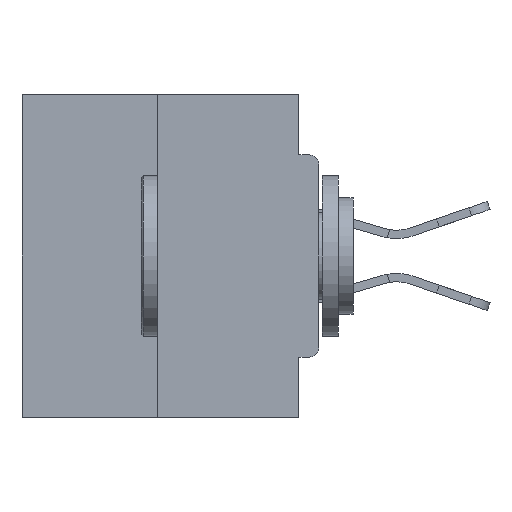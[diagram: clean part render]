
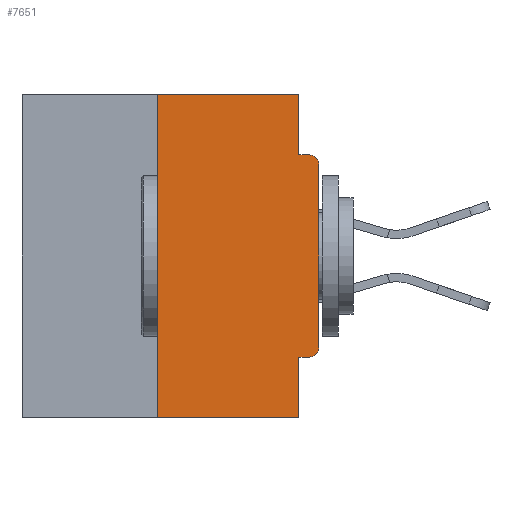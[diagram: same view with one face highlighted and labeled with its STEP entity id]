
A CAD part, left-side view. The second image highlights one B-rep face of the part: STEP entity #7651.
In plain terms, the highlighted planar face has unit normal (-1, 0, 0).
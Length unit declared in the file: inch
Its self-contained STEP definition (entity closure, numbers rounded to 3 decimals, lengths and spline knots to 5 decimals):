
#301 = FACE_OUTER_BOUND ( 'NONE', #33683, .T. ) ;
#410 = ORIENTED_EDGE ( 'NONE', *, *, #1086, .T. ) ;
#1086 = EDGE_CURVE ( 'NONE', #6244, #31713, #26061, .T. ) ;
#1896 = CARTESIAN_POINT ( 'NONE',  ( 0., 0., -0.0935 ) ) ;
#2441 = VERTEX_POINT ( 'NONE', #15004 ) ;
#2601 = CARTESIAN_POINT ( 'NONE',  ( 0., 0.015, -0.3915 ) ) ;
#3044 = DIRECTION ( 'NONE',  ( 0., 0., -1. ) ) ;
#3548 = CARTESIAN_POINT ( 'NONE',  ( 0., 0.46, -0.5 ) ) ;
#3959 = VECTOR ( 'NONE', #20573, 39.37008 ) ;
#4343 = VERTEX_POINT ( 'NONE', #19120 ) ;
#4525 = EDGE_CURVE ( 'NONE', #5938, #28625, #33759, .T. ) ;
#4541 = ORIENTED_EDGE ( 'NONE', *, *, #6182, .F. ) ;
#4792 = ORIENTED_EDGE ( 'NONE', *, *, #29375, .T. ) ;
#4930 = DIRECTION ( 'NONE',  ( 0., -1., 0. ) ) ;
#5081 = CARTESIAN_POINT ( 'NONE',  ( 0., 0., -0.4065 ) ) ;
#5479 = DIRECTION ( 'NONE',  ( 0., 0., 1. ) ) ;
#5938 = VERTEX_POINT ( 'NONE', #21699 ) ;
#6148 = ORIENTED_EDGE ( 'NONE', *, *, #4525, .F. ) ;
#6182 = EDGE_CURVE ( 'NONE', #21148, #2441, #33446, .T. ) ;
#6244 = VERTEX_POINT ( 'NONE', #33620 ) ;
#6263 = DIRECTION ( 'NONE',  ( 0., -1., 0. ) ) ;
#6662 = DIRECTION ( 'NONE',  ( 0., 0., -1. ) ) ;
#7127 = VECTOR ( 'NONE', #25434, 39.37008 ) ;
#7491 = CARTESIAN_POINT ( 'NONE',  ( 0., 0.46, 0. ) ) ;
#7647 = LINE ( 'NONE', #5081, #33552 ) ;
#7651 = ADVANCED_FACE ( 'NONE', ( #301 ), #21540, .F. ) ;
#7910 = DIRECTION ( 'NONE',  ( 0., 0., -1. ) ) ;
#8255 = VERTEX_POINT ( 'NONE', #18922 ) ;
#9831 = AXIS2_PLACEMENT_3D ( 'NONE', #2601, #31924, #3044 ) ;
#10408 = VECTOR ( 'NONE', #25734, 39.37008 ) ;
#10697 = AXIS2_PLACEMENT_3D ( 'NONE', #29740, #26821, #7910 ) ;
#11206 = CARTESIAN_POINT ( 'NONE',  ( 0., 0.25, -0.5 ) ) ;
#11615 = LINE ( 'NONE', #3548, #24999 ) ;
#12082 = VECTOR ( 'NONE', #4930, 39.37008 ) ;
#12343 = LINE ( 'NONE', #26829, #29495 ) ;
#13409 = ORIENTED_EDGE ( 'NONE', *, *, #32780, .T. ) ;
#13721 = CARTESIAN_POINT ( 'NONE',  ( 0., 0., -0.1085 ) ) ;
#14097 = VECTOR ( 'NONE', #6662, 39.37008 ) ;
#14639 = CARTESIAN_POINT ( 'NONE',  ( 0., 0.015, -0.1085 ) ) ;
#14680 = CARTESIAN_POINT ( 'NONE',  ( 0., 0.031, -0.5 ) ) ;
#15004 = CARTESIAN_POINT ( 'NONE',  ( 0., 0.031, -0.5 ) ) ;
#15741 = EDGE_CURVE ( 'NONE', #28625, #8255, #25265, .T. ) ;
#16924 = CARTESIAN_POINT ( 'NONE',  ( 0., 0.031, -0.4065 ) ) ;
#18922 = CARTESIAN_POINT ( 'NONE',  ( 0., 0.015, -0.0935 ) ) ;
#19120 = CARTESIAN_POINT ( 'NONE',  ( 0., 0.25, 0. ) ) ;
#19756 = CARTESIAN_POINT ( 'NONE',  ( 0., 0., 0. ) ) ;
#20026 = LINE ( 'NONE', #7491, #12082 ) ;
#20230 = CARTESIAN_POINT ( 'NONE',  ( 0., 0., -0.3915 ) ) ;
#20432 = LINE ( 'NONE', #19756, #10408 ) ;
#20573 = DIRECTION ( 'NONE',  ( 0., -1., 0. ) ) ;
#20821 = DIRECTION ( 'NONE',  ( 0., 1., 0. ) ) ;
#21148 = VERTEX_POINT ( 'NONE', #16924 ) ;
#21272 = AXIS2_PLACEMENT_3D ( 'NONE', #14639, #28099, #27875 ) ;
#21540 = PLANE ( 'NONE',  #10697 ) ;
#21699 = CARTESIAN_POINT ( 'NONE',  ( 0., 0.031, 0. ) ) ;
#22610 = ORIENTED_EDGE ( 'NONE', *, *, #31809, .F. ) ;
#23026 = ORIENTED_EDGE ( 'NONE', *, *, #30180, .F. ) ;
#24727 = ORIENTED_EDGE ( 'NONE', *, *, #15741, .F. ) ;
#24999 = VECTOR ( 'NONE', #6263, 39.37008 ) ;
#25265 = LINE ( 'NONE', #1896, #3959 ) ;
#25434 = DIRECTION ( 'NONE',  ( 0., 0., -1. ) ) ;
#25734 = DIRECTION ( 'NONE',  ( 0., 0., 1. ) ) ;
#26061 = CIRCLE ( 'NONE', #9831, 0.015 ) ;
#26821 = DIRECTION ( 'NONE',  ( 1., 0., 0. ) ) ;
#26829 = CARTESIAN_POINT ( 'NONE',  ( 0., 0.25, 0. ) ) ;
#27376 = CARTESIAN_POINT ( 'NONE',  ( 0., 0.031, -0.0935 ) ) ;
#27392 = VERTEX_POINT ( 'NONE', #13721 ) ;
#27744 = ORIENTED_EDGE ( 'NONE', *, *, #33617, .F. ) ;
#27875 = DIRECTION ( 'NONE',  ( 0., 0., -1. ) ) ;
#27990 = VERTEX_POINT ( 'NONE', #11206 ) ;
#28099 = DIRECTION ( 'NONE',  ( -1., 0., 0. ) ) ;
#28625 = VERTEX_POINT ( 'NONE', #27376 ) ;
#28774 = EDGE_CURVE ( 'NONE', #31713, #27392, #20432, .T. ) ;
#28916 = CIRCLE ( 'NONE', #21272, 0.015 ) ;
#29375 = EDGE_CURVE ( 'NONE', #27990, #2441, #11615, .T. ) ;
#29495 = VECTOR ( 'NONE', #5479, 39.37008 ) ;
#29740 = CARTESIAN_POINT ( 'NONE',  ( 0., 0.46, 0. ) ) ;
#30180 = EDGE_CURVE ( 'NONE', #27990, #4343, #12343, .T. ) ;
#31713 = VERTEX_POINT ( 'NONE', #20230 ) ;
#31809 = EDGE_CURVE ( 'NONE', #6244, #21148, #7647, .T. ) ;
#31924 = DIRECTION ( 'NONE',  ( -1., 0., 0. ) ) ;
#32780 = EDGE_CURVE ( 'NONE', #27392, #8255, #28916, .T. ) ;
#33047 = CARTESIAN_POINT ( 'NONE',  ( 0., 0.031, 0. ) ) ;
#33446 = LINE ( 'NONE', #14680, #7127 ) ;
#33552 = VECTOR ( 'NONE', #20821, 39.37008 ) ;
#33617 = EDGE_CURVE ( 'NONE', #4343, #5938, #20026, .T. ) ;
#33620 = CARTESIAN_POINT ( 'NONE',  ( 0., 0.015, -0.4065 ) ) ;
#33683 = EDGE_LOOP ( 'NONE', ( #27744, #23026, #4792, #4541, #22610, #410, #34621, #13409, #24727, #6148 ) ) ;
#33759 = LINE ( 'NONE', #33047, #14097 ) ;
#34621 = ORIENTED_EDGE ( 'NONE', *, *, #28774, .T. ) ;
